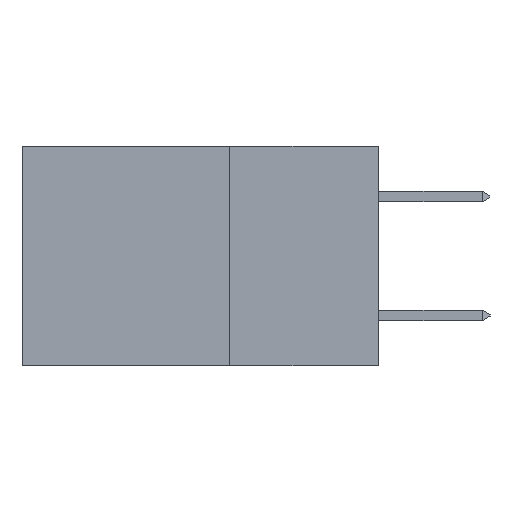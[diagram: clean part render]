
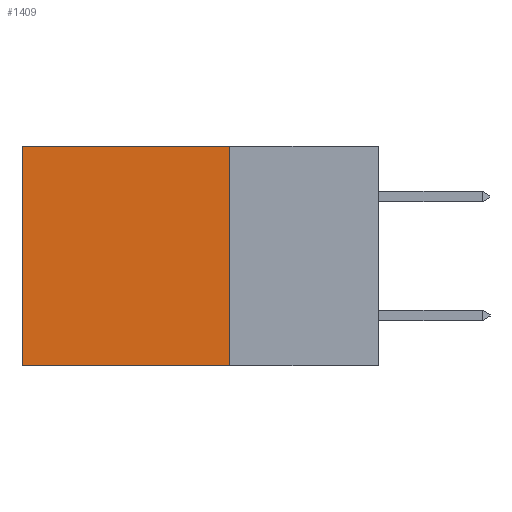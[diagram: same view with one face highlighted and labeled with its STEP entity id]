
A CAD part, left-side view. The second image highlights one B-rep face of the part: STEP entity #1409.
In plain terms, the highlighted planar face has unit normal (-1, 0, 0).
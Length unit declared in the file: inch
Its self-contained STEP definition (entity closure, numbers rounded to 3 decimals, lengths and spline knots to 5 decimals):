
#128 = DIRECTION ( 'NONE',  ( 0., 1., 0. ) ) ;
#178 = LINE ( 'NONE', #5678, #5296 ) ;
#215 = CARTESIAN_POINT ( 'NONE',  ( 0.2615, 0.25, 0. ) ) ;
#464 = PLANE ( 'NONE',  #6387 ) ;
#1346 = VECTOR ( 'NONE', #4954, 39.37008 ) ;
#1409 = ADVANCED_FACE ( 'NONE', ( #7844 ), #464, .F. ) ;
#1990 = VERTEX_POINT ( 'NONE', #5681 ) ;
#2261 = EDGE_LOOP ( 'NONE', ( #3142, #3174, #4435, #4637 ) ) ;
#3142 = ORIENTED_EDGE ( 'NONE', *, *, #5193, .T. ) ;
#3174 = ORIENTED_EDGE ( 'NONE', *, *, #6283, .F. ) ;
#3437 = LINE ( 'NONE', #215, #8337 ) ;
#3640 = CARTESIAN_POINT ( 'NONE',  ( 0.2615, 0.25, 0. ) ) ;
#4435 = ORIENTED_EDGE ( 'NONE', *, *, #6220, .F. ) ;
#4637 = ORIENTED_EDGE ( 'NONE', *, *, #4956, .T. ) ;
#4751 = CARTESIAN_POINT ( 'NONE',  ( 0.2615, 0.25, -0.37 ) ) ;
#4773 = DIRECTION ( 'NONE',  ( 0., 1., 0. ) ) ;
#4876 = DIRECTION ( 'NONE',  ( 0., 0., -1. ) ) ;
#4954 = DIRECTION ( 'NONE',  ( 0., 0., -1. ) ) ;
#4956 = EDGE_CURVE ( 'NONE', #6483, #1990, #3437, .T. ) ;
#4990 = LINE ( 'NONE', #5001, #1346 ) ;
#5001 = CARTESIAN_POINT ( 'NONE',  ( 0.2615, 0.25, -0.37 ) ) ;
#5193 = EDGE_CURVE ( 'NONE', #1990, #8379, #178, .T. ) ;
#5296 = VECTOR ( 'NONE', #5624, 39.37008 ) ;
#5624 = DIRECTION ( 'NONE',  ( 0., 0., -1. ) ) ;
#5678 = CARTESIAN_POINT ( 'NONE',  ( 0.2615, 0.6, -0.37 ) ) ;
#5681 = CARTESIAN_POINT ( 'NONE',  ( 0.2615, 0.6, 0. ) ) ;
#6220 = EDGE_CURVE ( 'NONE', #6483, #8341, #4990, .T. ) ;
#6283 = EDGE_CURVE ( 'NONE', #8341, #8379, #7953, .T. ) ;
#6387 = AXIS2_PLACEMENT_3D ( 'NONE', #7751, #6537, #4876 ) ;
#6480 = VECTOR ( 'NONE', #4773, 39.37008 ) ;
#6483 = VERTEX_POINT ( 'NONE', #3640 ) ;
#6537 = DIRECTION ( 'NONE',  ( 1., 0., 0. ) ) ;
#7751 = CARTESIAN_POINT ( 'NONE',  ( 0.2615, 0.25, -0.37 ) ) ;
#7844 = FACE_OUTER_BOUND ( 'NONE', #2261, .T. ) ;
#7907 = CARTESIAN_POINT ( 'NONE',  ( 0.2615, 0.25, -0.37 ) ) ;
#7926 = CARTESIAN_POINT ( 'NONE',  ( 0.2615, 0.6, -0.37 ) ) ;
#7953 = LINE ( 'NONE', #4751, #6480 ) ;
#8337 = VECTOR ( 'NONE', #128, 39.37008 ) ;
#8341 = VERTEX_POINT ( 'NONE', #7907 ) ;
#8379 = VERTEX_POINT ( 'NONE', #7926 ) ;
